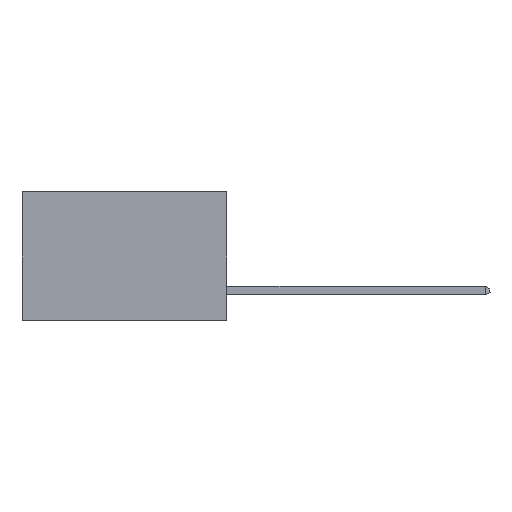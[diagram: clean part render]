
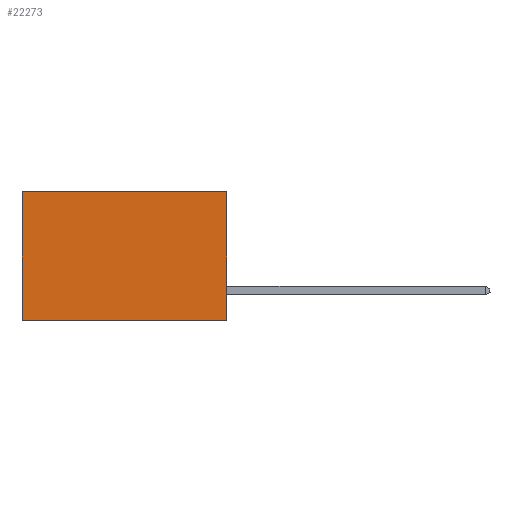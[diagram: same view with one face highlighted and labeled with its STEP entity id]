
A CAD part, left-side view. The second image highlights one B-rep face of the part: STEP entity #22273.
In plain terms, the highlighted planar face has unit normal (-1, 0, 0).
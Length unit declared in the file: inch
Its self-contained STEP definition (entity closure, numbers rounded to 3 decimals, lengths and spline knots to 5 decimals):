
#177 = VERTEX_POINT ( 'NONE', #10852 ) ;
#345 = CARTESIAN_POINT ( 'NONE',  ( 0.277, 0.59, -0.37 ) ) ;
#614 = DIRECTION ( 'NONE',  ( 0., 0., -1. ) ) ;
#706 = LINE ( 'NONE', #22834, #5021 ) ;
#2003 = EDGE_CURVE ( 'NONE', #8432, #11083, #3618, .T. ) ;
#2132 = LINE ( 'NONE', #16376, #6450 ) ;
#2923 = CARTESIAN_POINT ( 'NONE',  ( 0.277, 0., -0.37 ) ) ;
#3120 = DIRECTION ( 'NONE',  ( 0., 0., -1. ) ) ;
#3618 = LINE ( 'NONE', #6715, #23035 ) ;
#5021 = VECTOR ( 'NONE', #8357, 39.37008 ) ;
#5083 = ORIENTED_EDGE ( 'NONE', *, *, #2003, .F. ) ;
#6450 = VECTOR ( 'NONE', #10943, 39.37008 ) ;
#6715 = CARTESIAN_POINT ( 'NONE',  ( 0.277, 0., -0.37 ) ) ;
#7441 = VERTEX_POINT ( 'NONE', #345 ) ;
#8357 = DIRECTION ( 'NONE',  ( 0., 1., 0. ) ) ;
#8432 = VERTEX_POINT ( 'NONE', #12246 ) ;
#9344 = ORIENTED_EDGE ( 'NONE', *, *, #16794, .F. ) ;
#9366 = LINE ( 'NONE', #9803, #23283 ) ;
#9803 = CARTESIAN_POINT ( 'NONE',  ( 0.277, 0.59, -0.37 ) ) ;
#10852 = CARTESIAN_POINT ( 'NONE',  ( 0.277, 0.59, 0. ) ) ;
#10943 = DIRECTION ( 'NONE',  ( 0., 1., 0. ) ) ;
#11083 = VERTEX_POINT ( 'NONE', #2923 ) ;
#12246 = CARTESIAN_POINT ( 'NONE',  ( 0.277, 0., 0. ) ) ;
#12301 = PLANE ( 'NONE',  #14391 ) ;
#13941 = ORIENTED_EDGE ( 'NONE', *, *, #14804, .T. ) ;
#14046 = ORIENTED_EDGE ( 'NONE', *, *, #16650, .T. ) ;
#14135 = DIRECTION ( 'NONE',  ( 1., 0., 0. ) ) ;
#14391 = AXIS2_PLACEMENT_3D ( 'NONE', #23127, #14135, #3120 ) ;
#14804 = EDGE_CURVE ( 'NONE', #177, #7441, #9366, .T. ) ;
#16135 = DIRECTION ( 'NONE',  ( 0., 0., -1. ) ) ;
#16376 = CARTESIAN_POINT ( 'NONE',  ( 0.277, 0., -0.37 ) ) ;
#16650 = EDGE_CURVE ( 'NONE', #8432, #177, #706, .T. ) ;
#16794 = EDGE_CURVE ( 'NONE', #11083, #7441, #2132, .T. ) ;
#19446 = FACE_OUTER_BOUND ( 'NONE', #21768, .T. ) ;
#21768 = EDGE_LOOP ( 'NONE', ( #13941, #9344, #5083, #14046 ) ) ;
#22273 = ADVANCED_FACE ( 'NONE', ( #19446 ), #12301, .F. ) ;
#22834 = CARTESIAN_POINT ( 'NONE',  ( 0.277, 0., 0. ) ) ;
#23035 = VECTOR ( 'NONE', #16135, 39.37008 ) ;
#23127 = CARTESIAN_POINT ( 'NONE',  ( 0.277, 0., -0.37 ) ) ;
#23283 = VECTOR ( 'NONE', #614, 39.37008 ) ;
